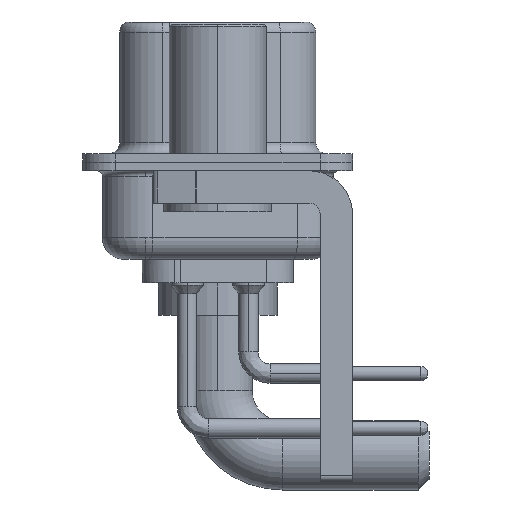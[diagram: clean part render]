
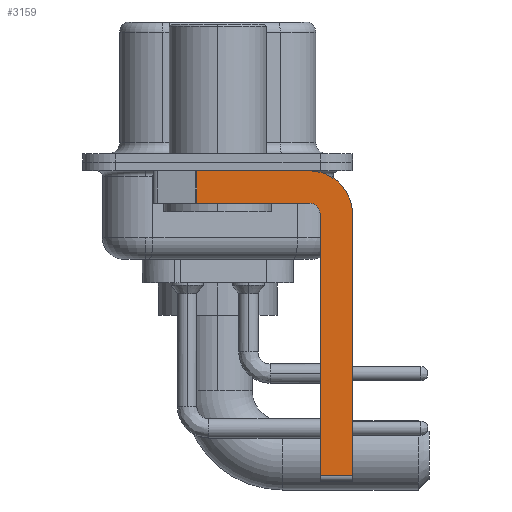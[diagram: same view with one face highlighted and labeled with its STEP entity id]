
A CAD part, left-side view. The second image highlights one B-rep face of the part: STEP entity #3159.
In plain terms, the highlighted planar face has unit normal (-1, 0, 0).
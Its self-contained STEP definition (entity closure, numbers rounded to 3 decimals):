
#3 = CARTESIAN_POINT ( 'NONE',  ( -2.9, -6.25, -2.4 ) ) ;
#72 = LINE ( 'NONE', #19066, #17322 ) ;
#534 = CARTESIAN_POINT ( 'NONE',  ( -2.9, 0.978, -1.9 ) ) ;
#805 = EDGE_CURVE ( 'NONE', #24129, #7646, #14582, .T. ) ;
#1182 = EDGE_CURVE ( 'NONE', #2926, #5517, #9159, .T. ) ;
#1456 = ORIENTED_EDGE ( 'NONE', *, *, #6230, .F. ) ;
#1714 = ORIENTED_EDGE ( 'NONE', *, *, #18420, .F. ) ;
#2499 = CARTESIAN_POINT ( 'NONE',  ( -2.9, -4.25, -2.4 ) ) ;
#2917 = VECTOR ( 'NONE', #5346, 1000. ) ;
#2926 = VERTEX_POINT ( 'NONE', #9767 ) ;
#3159 = ADVANCED_FACE ( 'NONE', ( #22212 ), #6727, .F. ) ;
#3619 = DIRECTION ( 'NONE',  ( 0., 0., 1. ) ) ;
#4901 = CARTESIAN_POINT ( 'NONE',  ( -2.9, 0.978, -1.9 ) ) ;
#5346 = DIRECTION ( 'NONE',  ( 0., -1., 0. ) ) ;
#5517 = VERTEX_POINT ( 'NONE', #3 ) ;
#5722 = DIRECTION ( 'NONE',  ( 0., -1., 0. ) ) ;
#6230 = EDGE_CURVE ( 'NONE', #24129, #2926, #8598, .T. ) ;
#6727 = PLANE ( 'NONE',  #6808 ) ;
#6808 = AXIS2_PLACEMENT_3D ( 'NONE', #22335, #10514, #8729 ) ;
#6881 = CARTESIAN_POINT ( 'NONE',  ( -2.9, -4.25, -1.9 ) ) ;
#7264 = LINE ( 'NONE', #13056, #24105 ) ;
#7646 = VERTEX_POINT ( 'NONE', #534 ) ;
#8270 = DIRECTION ( 'NONE',  ( 0., 0., -1. ) ) ;
#8310 = CARTESIAN_POINT ( 'NONE',  ( -2.9, -4.75, -14.55 ) ) ;
#8434 = ORIENTED_EDGE ( 'NONE', *, *, #1182, .F. ) ;
#8598 = LINE ( 'NONE', #16787, #2917 ) ;
#8729 = DIRECTION ( 'NONE',  ( 0., 0., -1. ) ) ;
#8742 = AXIS2_PLACEMENT_3D ( 'NONE', #2499, #17843, #8270 ) ;
#9001 = LINE ( 'NONE', #6881, #9266 ) ;
#9012 = CARTESIAN_POINT ( 'NONE',  ( -2.9, -6.25, -2.4 ) ) ;
#9159 = CIRCLE ( 'NONE', #8742, 2. ) ;
#9266 = VECTOR ( 'NONE', #16317, 1000. ) ;
#9576 = CARTESIAN_POINT ( 'NONE',  ( -2.9, -6.25, -14.55 ) ) ;
#9767 = CARTESIAN_POINT ( 'NONE',  ( -2.9, -4.25, -0.4 ) ) ;
#10046 = AXIS2_PLACEMENT_3D ( 'NONE', #18293, #24102, #22700 ) ;
#10514 = DIRECTION ( 'NONE',  ( 1., 0., 0. ) ) ;
#11598 = ORIENTED_EDGE ( 'NONE', *, *, #17415, .F. ) ;
#12050 = VERTEX_POINT ( 'NONE', #9576 ) ;
#12445 = CIRCLE ( 'NONE', #10046, 0.5 ) ;
#13056 = CARTESIAN_POINT ( 'NONE',  ( -2.9, -4.75, -14.8 ) ) ;
#13406 = VERTEX_POINT ( 'NONE', #14960 ) ;
#13442 = ORIENTED_EDGE ( 'NONE', *, *, #20375, .T. ) ;
#14582 = LINE ( 'NONE', #4901, #23252 ) ;
#14658 = ORIENTED_EDGE ( 'NONE', *, *, #805, .T. ) ;
#14960 = CARTESIAN_POINT ( 'NONE',  ( -2.9, -4.25, -1.9 ) ) ;
#16317 = DIRECTION ( 'NONE',  ( 0., 1., 0. ) ) ;
#16787 = CARTESIAN_POINT ( 'NONE',  ( -2.9, 3., -0.4 ) ) ;
#17133 = EDGE_CURVE ( 'NONE', #20987, #21719, #7264, .T. ) ;
#17322 = VECTOR ( 'NONE', #5722, 1000. ) ;
#17415 = EDGE_CURVE ( 'NONE', #21719, #13406, #12445, .T. ) ;
#17518 = ORIENTED_EDGE ( 'NONE', *, *, #17133, .F. ) ;
#17843 = DIRECTION ( 'NONE',  ( 1., 0., 0. ) ) ;
#18104 = LINE ( 'NONE', #9012, #20615 ) ;
#18293 = CARTESIAN_POINT ( 'NONE',  ( -2.9, -4.25, -2.4 ) ) ;
#18420 = EDGE_CURVE ( 'NONE', #13406, #7646, #9001, .T. ) ;
#18545 = EDGE_LOOP ( 'NONE', ( #1456, #14658, #1714, #11598, #17518, #13442, #19564, #8434 ) ) ;
#19066 = CARTESIAN_POINT ( 'NONE',  ( -2.9, -4.25, -14.55 ) ) ;
#19564 = ORIENTED_EDGE ( 'NONE', *, *, #22399, .F. ) ;
#20375 = EDGE_CURVE ( 'NONE', #20987, #12050, #72, .T. ) ;
#20607 = CARTESIAN_POINT ( 'NONE',  ( -2.9, -4.75, -2.4 ) ) ;
#20615 = VECTOR ( 'NONE', #23906, 1000. ) ;
#20987 = VERTEX_POINT ( 'NONE', #8310 ) ;
#21719 = VERTEX_POINT ( 'NONE', #20607 ) ;
#22212 = FACE_OUTER_BOUND ( 'NONE', #18545, .T. ) ;
#22271 = DIRECTION ( 'NONE',  ( 0., 0., -1. ) ) ;
#22335 = CARTESIAN_POINT ( 'NONE',  ( -2.9, -4.25, -2.4 ) ) ;
#22399 = EDGE_CURVE ( 'NONE', #5517, #12050, #18104, .T. ) ;
#22700 = DIRECTION ( 'NONE',  ( 0., 0., 1. ) ) ;
#23252 = VECTOR ( 'NONE', #22271, 1000. ) ;
#23906 = DIRECTION ( 'NONE',  ( 0., 0., -1. ) ) ;
#24102 = DIRECTION ( 'NONE',  ( -1., 0., 0. ) ) ;
#24105 = VECTOR ( 'NONE', #3619, 1000. ) ;
#24129 = VERTEX_POINT ( 'NONE', #24372 ) ;
#24372 = CARTESIAN_POINT ( 'NONE',  ( -2.9, 0.978, -0.4 ) ) ;
